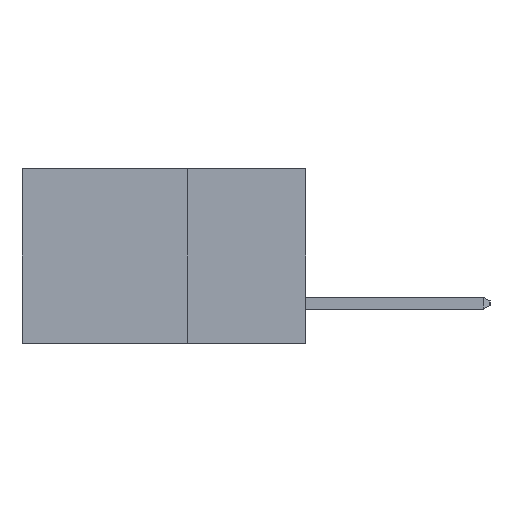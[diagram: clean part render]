
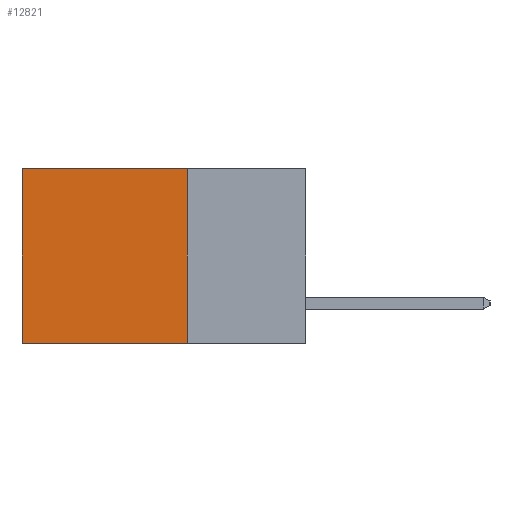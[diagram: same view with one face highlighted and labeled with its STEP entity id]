
A CAD part, left-side view. The second image highlights one B-rep face of the part: STEP entity #12821.
In plain terms, the highlighted planar face has unit normal (-1, 0, 0).
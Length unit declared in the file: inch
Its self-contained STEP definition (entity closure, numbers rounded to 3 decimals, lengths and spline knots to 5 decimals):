
#45 = VECTOR ( 'NONE', #2938, 39.37008 ) ;
#656 = LINE ( 'NONE', #4843, #45 ) ;
#1422 = DIRECTION ( 'NONE',  ( 1., 0., 0. ) ) ;
#1569 = VERTEX_POINT ( 'NONE', #10070 ) ;
#2558 = CARTESIAN_POINT ( 'NONE',  ( 0.298, 0.25, 0. ) ) ;
#2938 = DIRECTION ( 'NONE',  ( 0., 0., -1. ) ) ;
#4676 = VERTEX_POINT ( 'NONE', #16888 ) ;
#4843 = CARTESIAN_POINT ( 'NONE',  ( 0.298, 0.6, 0. ) ) ;
#7056 = ORIENTED_EDGE ( 'NONE', *, *, #15751, .F. ) ;
#8813 = ORIENTED_EDGE ( 'NONE', *, *, #11439, .T. ) ;
#9128 = CARTESIAN_POINT ( 'NONE',  ( 0.298, 0.25, 0. ) ) ;
#9436 = CARTESIAN_POINT ( 'NONE',  ( 0.298, 0.6, 0. ) ) ;
#10070 = CARTESIAN_POINT ( 'NONE',  ( 0.298, 0.6, -0.37 ) ) ;
#10072 = DIRECTION ( 'NONE',  ( 0., 1., 0. ) ) ;
#11349 = VECTOR ( 'NONE', #16982, 39.37008 ) ;
#11439 = EDGE_CURVE ( 'NONE', #11686, #1569, #656, .T. ) ;
#11686 = VERTEX_POINT ( 'NONE', #9436 ) ;
#12455 = ORIENTED_EDGE ( 'NONE', *, *, #24320, .F. ) ;
#12821 = ADVANCED_FACE ( 'NONE', ( #12950 ), #12957, .F. ) ;
#12950 = FACE_OUTER_BOUND ( 'NONE', #15168, .T. ) ;
#12957 = PLANE ( 'NONE',  #22561 ) ;
#13116 = DIRECTION ( 'NONE',  ( 0., 1., 0. ) ) ;
#14850 = DIRECTION ( 'NONE',  ( 0., 0., -1. ) ) ;
#14901 = LINE ( 'NONE', #17661, #19239 ) ;
#14920 = CARTESIAN_POINT ( 'NONE',  ( 0.298, 0.25, 0. ) ) ;
#15103 = CARTESIAN_POINT ( 'NONE',  ( 0.298, 0.25, 0. ) ) ;
#15168 = EDGE_LOOP ( 'NONE', ( #8813, #12455, #7056, #19944 ) ) ;
#15751 = EDGE_CURVE ( 'NONE', #17000, #4676, #16970, .T. ) ;
#16029 = LINE ( 'NONE', #14920, #20332 ) ;
#16888 = CARTESIAN_POINT ( 'NONE',  ( 0.298, 0.25, -0.37 ) ) ;
#16970 = LINE ( 'NONE', #15103, #11349 ) ;
#16982 = DIRECTION ( 'NONE',  ( 0., 0., -1. ) ) ;
#17000 = VERTEX_POINT ( 'NONE', #2558 ) ;
#17661 = CARTESIAN_POINT ( 'NONE',  ( 0.298, 0.25, -0.37 ) ) ;
#19239 = VECTOR ( 'NONE', #10072, 39.37008 ) ;
#19944 = ORIENTED_EDGE ( 'NONE', *, *, #20388, .T. ) ;
#20332 = VECTOR ( 'NONE', #13116, 39.37008 ) ;
#20388 = EDGE_CURVE ( 'NONE', #17000, #11686, #16029, .T. ) ;
#22561 = AXIS2_PLACEMENT_3D ( 'NONE', #9128, #1422, #14850 ) ;
#24320 = EDGE_CURVE ( 'NONE', #4676, #1569, #14901, .T. ) ;
